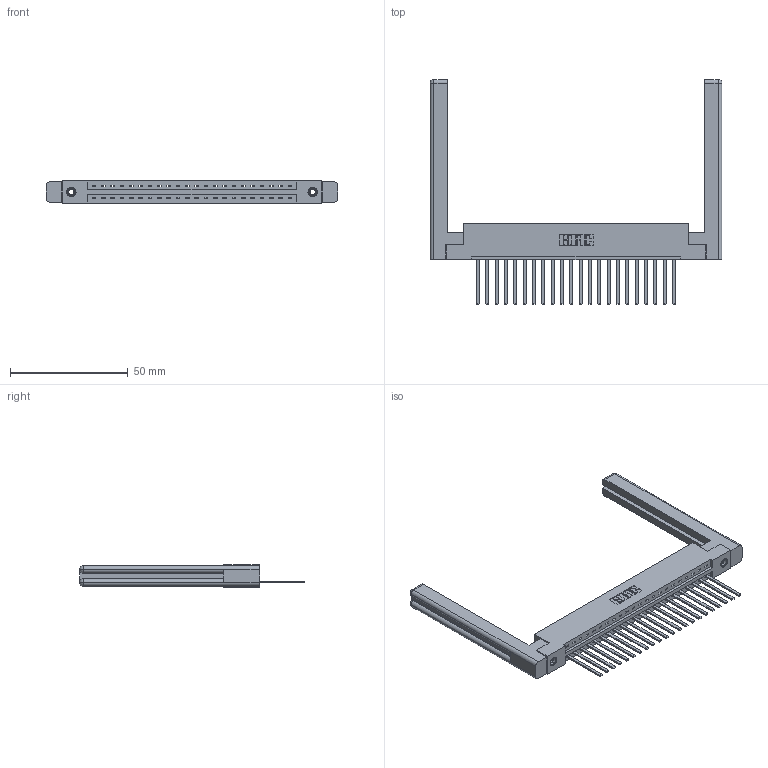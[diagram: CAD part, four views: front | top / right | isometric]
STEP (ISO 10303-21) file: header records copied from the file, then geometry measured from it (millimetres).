
FILE_DESCRIPTION (( 'STEP AP203' ), '1' );
FILE_NAME ('337-022-544-158.STEP', '2019-09-30T14:00:47', ( '' ), ( '' ), 'SwSTEP 2.0', 'SolidWorks 2016', '' );
FILE_SCHEMA (( 'CONFIG_CONTROL_DESIGN' ));
Length unit declared in the file: inch
Products named in the file (5): 337-022-544-158; 307-220-058; 345-292-001_345-293-144; 345-250-001_345-250-001-102; 337 Part_Flush Mounting Lugs - 0.156 Dia-TI
Assembly tree (27 placements, depth 2):
  337-022-544-158
    337 Part_Flush Mounting Lugs - 0.156 Dia-TI
    345-292-001_345-293-144  x22
    345-250-001_345-250-001-102  x2
    307-220-058  x2
Bounding box: 123.8 x 95.38 x 9.4 mm (x, y, z)
Volume: 20033.6 mm3; surface area: 19240.9 mm2
Topology: 27 solids, 27 shells, 1488 faces, 4405 edges, 2894 vertices
Faces by surface type: plane 1078, cylinder 386, cone 12, torus 12
Entity records: 21390 total; most frequent: CARTESIAN_POINT 3723, ORIENTED_EDGE 3620, DIRECTION 3190, EDGE_CURVE 1810, LINE 1638, VECTOR 1638, VERTEX_POINT 1198, AXIS2_PLACEMENT_3D 776
